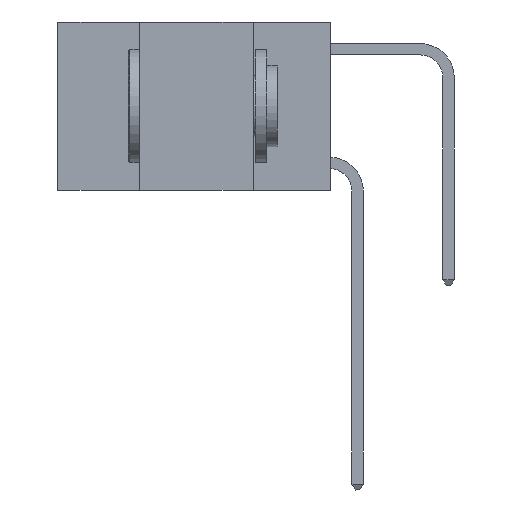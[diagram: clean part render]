
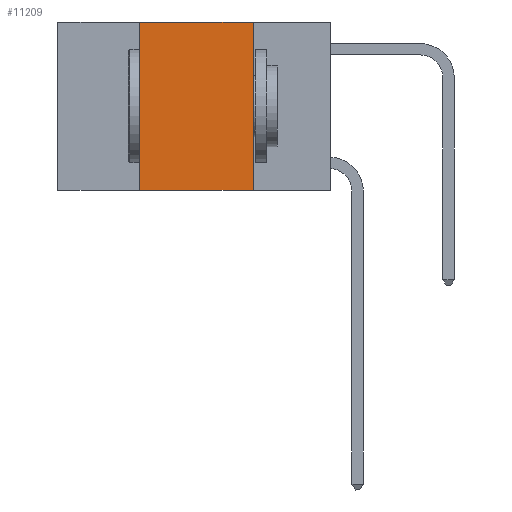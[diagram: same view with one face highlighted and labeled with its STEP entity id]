
A CAD part, left-side view. The second image highlights one B-rep face of the part: STEP entity #11209.
In plain terms, the highlighted planar face has unit normal (-1, 0, 0).
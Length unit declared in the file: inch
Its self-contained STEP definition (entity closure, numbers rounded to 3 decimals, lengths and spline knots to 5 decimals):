
#717 = CARTESIAN_POINT ( 'NONE',  ( 0., 0.17, 0. ) ) ;
#1348 = CARTESIAN_POINT ( 'NONE',  ( 0., 0.42, 0. ) ) ;
#1573 = VECTOR ( 'NONE', #8535, 39.37008 ) ;
#1748 = CARTESIAN_POINT ( 'NONE',  ( 0., 0.17, 0. ) ) ;
#2637 = LINE ( 'NONE', #14174, #1573 ) ;
#2760 = VECTOR ( 'NONE', #12748, 39.37008 ) ;
#3049 = EDGE_CURVE ( 'NONE', #12094, #7825, #9677, .T. ) ;
#3212 = ORIENTED_EDGE ( 'NONE', *, *, #9742, .T. ) ;
#3397 = ORIENTED_EDGE ( 'NONE', *, *, #12860, .F. ) ;
#3402 = CARTESIAN_POINT ( 'NONE',  ( 0., 0.6, 0. ) ) ;
#3832 = CARTESIAN_POINT ( 'NONE',  ( 0., 0.6, -0.37 ) ) ;
#4965 = LINE ( 'NONE', #3832, #9268 ) ;
#6776 = CARTESIAN_POINT ( 'NONE',  ( 0., 0.42, 0. ) ) ;
#7478 = ORIENTED_EDGE ( 'NONE', *, *, #3049, .F. ) ;
#7825 = VERTEX_POINT ( 'NONE', #13040 ) ;
#8040 = DIRECTION ( 'NONE',  ( 1., 0., 0. ) ) ;
#8440 = DIRECTION ( 'NONE',  ( 0., -1., 0. ) ) ;
#8535 = DIRECTION ( 'NONE',  ( 0., -1., 0. ) ) ;
#9052 = EDGE_LOOP ( 'NONE', ( #7478, #3397, #11204, #3212 ) ) ;
#9070 = FACE_OUTER_BOUND ( 'NONE', #9052, .T. ) ;
#9147 = PLANE ( 'NONE',  #10493 ) ;
#9268 = VECTOR ( 'NONE', #8440, 39.37008 ) ;
#9677 = LINE ( 'NONE', #717, #13656 ) ;
#9742 = EDGE_CURVE ( 'NONE', #14041, #7825, #4965, .T. ) ;
#10281 = EDGE_CURVE ( 'NONE', #14041, #13481, #10484, .T. ) ;
#10484 = LINE ( 'NONE', #1348, #2760 ) ;
#10493 = AXIS2_PLACEMENT_3D ( 'NONE', #3402, #8040, #12597 ) ;
#11204 = ORIENTED_EDGE ( 'NONE', *, *, #10281, .F. ) ;
#11209 = ADVANCED_FACE ( 'NONE', ( #9070 ), #9147, .F. ) ;
#12094 = VERTEX_POINT ( 'NONE', #1748 ) ;
#12597 = DIRECTION ( 'NONE',  ( 0., 0., -1. ) ) ;
#12748 = DIRECTION ( 'NONE',  ( 0., 0., 1. ) ) ;
#12860 = EDGE_CURVE ( 'NONE', #13481, #12094, #2637, .T. ) ;
#13040 = CARTESIAN_POINT ( 'NONE',  ( 0., 0.17, -0.37 ) ) ;
#13276 = DIRECTION ( 'NONE',  ( 0., 0., -1. ) ) ;
#13481 = VERTEX_POINT ( 'NONE', #6776 ) ;
#13656 = VECTOR ( 'NONE', #13276, 39.37008 ) ;
#13707 = CARTESIAN_POINT ( 'NONE',  ( 0., 0.42, -0.37 ) ) ;
#14041 = VERTEX_POINT ( 'NONE', #13707 ) ;
#14174 = CARTESIAN_POINT ( 'NONE',  ( 0., 0.6, 0. ) ) ;
